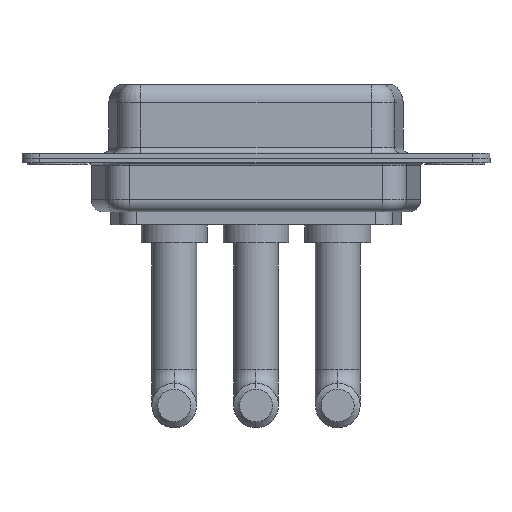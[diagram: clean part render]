
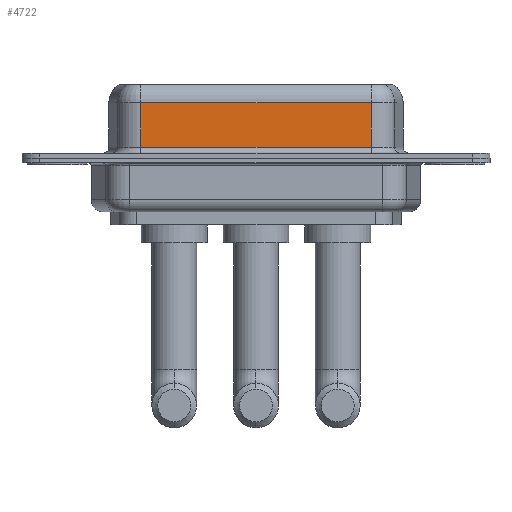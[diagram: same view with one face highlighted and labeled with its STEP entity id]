
A CAD part, front view. The second image highlights one B-rep face of the part: STEP entity #4722.
In plain terms, the highlighted planar face has unit normal (0, -1, 0).
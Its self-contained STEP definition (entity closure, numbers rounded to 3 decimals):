
#953 = VERTEX_POINT ( 'NONE', #10434 ) ;
#1164 = DIRECTION ( 'NONE',  ( 0., 0., -1. ) ) ;
#1255 = CARTESIAN_POINT ( 'NONE',  ( 26.287, -3.95, 6.4 ) ) ;
#1371 = ORIENTED_EDGE ( 'NONE', *, *, #2948, .F. ) ;
#1516 = VECTOR ( 'NONE', #3624, 1000. ) ;
#1784 = DIRECTION ( 'NONE',  ( -1., 0., 0. ) ) ;
#1839 = CARTESIAN_POINT ( 'NONE',  ( 26.287, -3.95, 4.65 ) ) ;
#1872 = VECTOR ( 'NONE', #1784, 1000. ) ;
#1974 = CARTESIAN_POINT ( 'NONE',  ( 26.287, -3.95, 6.4 ) ) ;
#2046 = VERTEX_POINT ( 'NONE', #4365 ) ;
#2816 = CARTESIAN_POINT ( 'NONE',  ( 26.287, -3.95, 0.9 ) ) ;
#2948 = EDGE_CURVE ( 'NONE', #953, #7098, #10095, .T. ) ;
#3624 = DIRECTION ( 'NONE',  ( 1., 0., 0. ) ) ;
#3719 = DIRECTION ( 'NONE',  ( 0., 1., 0. ) ) ;
#4365 = CARTESIAN_POINT ( 'NONE',  ( 7.013, -3.95, 4.65 ) ) ;
#4473 = PLANE ( 'NONE',  #5589 ) ;
#4586 = EDGE_CURVE ( 'NONE', #2046, #5767, #6661, .T. ) ;
#4722 = ADVANCED_FACE ( 'NONE', ( #6287 ), #4473, .F. ) ;
#5208 = VECTOR ( 'NONE', #1164, 1000. ) ;
#5589 = AXIS2_PLACEMENT_3D ( 'NONE', #1255, #3719, #6862 ) ;
#5767 = VERTEX_POINT ( 'NONE', #6602 ) ;
#5864 = EDGE_CURVE ( 'NONE', #5767, #7098, #7619, .T. ) ;
#6280 = ORIENTED_EDGE ( 'NONE', *, *, #4586, .T. ) ;
#6287 = FACE_OUTER_BOUND ( 'NONE', #6827, .T. ) ;
#6584 = LINE ( 'NONE', #1839, #1872 ) ;
#6602 = CARTESIAN_POINT ( 'NONE',  ( 7.013, -3.95, 0.9 ) ) ;
#6661 = LINE ( 'NONE', #7567, #8988 ) ;
#6827 = EDGE_LOOP ( 'NONE', ( #1371, #7071, #6280, #9060 ) ) ;
#6862 = DIRECTION ( 'NONE',  ( 0., 0., 1. ) ) ;
#7071 = ORIENTED_EDGE ( 'NONE', *, *, #7617, .T. ) ;
#7098 = VERTEX_POINT ( 'NONE', #8116 ) ;
#7567 = CARTESIAN_POINT ( 'NONE',  ( 7.013, -3.95, 6.4 ) ) ;
#7617 = EDGE_CURVE ( 'NONE', #953, #2046, #6584, .T. ) ;
#7619 = LINE ( 'NONE', #2816, #1516 ) ;
#8116 = CARTESIAN_POINT ( 'NONE',  ( 26.287, -3.95, 0.9 ) ) ;
#8988 = VECTOR ( 'NONE', #10029, 1000. ) ;
#9060 = ORIENTED_EDGE ( 'NONE', *, *, #5864, .T. ) ;
#10029 = DIRECTION ( 'NONE',  ( 0., 0., -1. ) ) ;
#10095 = LINE ( 'NONE', #1974, #5208 ) ;
#10434 = CARTESIAN_POINT ( 'NONE',  ( 26.287, -3.95, 4.65 ) ) ;
